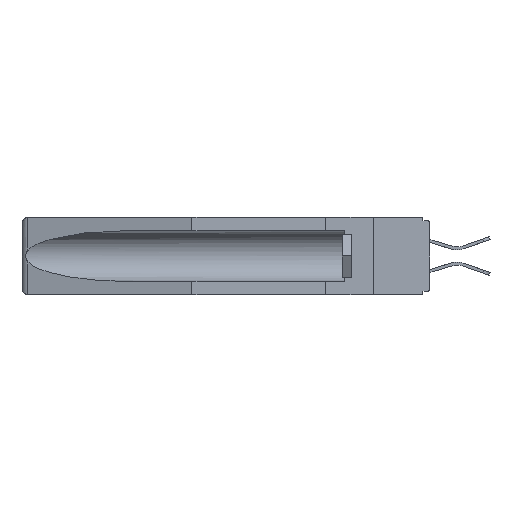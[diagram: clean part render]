
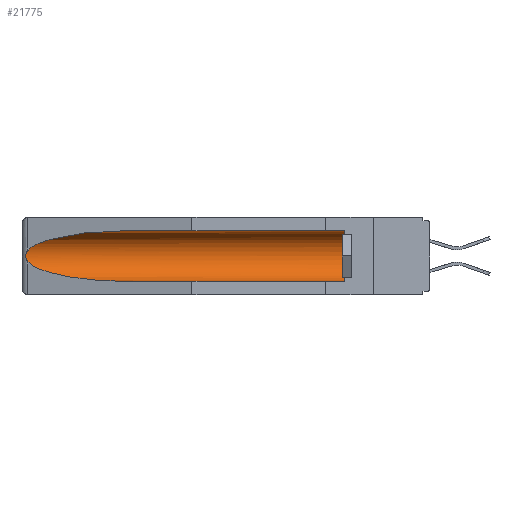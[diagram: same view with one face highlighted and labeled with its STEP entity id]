
A CAD part, left-side view. The second image highlights one B-rep face of the part: STEP entity #21775.
In plain terms, the highlighted cylindrical face has radius 2.857 mm (diameter 5.715 mm), a partial arc.
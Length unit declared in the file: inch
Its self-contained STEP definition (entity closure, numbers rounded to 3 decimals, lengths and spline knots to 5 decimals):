
#43 = CARTESIAN_POINT ( 'NONE',  ( 0.155, 1.07973, -0.284 ) ) ;
#302 = CARTESIAN_POINT ( 'NONE',  ( 0.155, 0.126, -0.284 ) ) ;
#772 = DIRECTION ( 'NONE',  ( 0., 1., 0. ) ) ;
#1684 = CARTESIAN_POINT ( 'NONE',  ( 0.155, 0.126, -0.059 ) ) ;
#1730 = DIRECTION ( 'NONE',  ( 0., 0., 1. ) ) ;
#1819 = CARTESIAN_POINT ( 'NONE',  ( 0.25451, 1.48313, -0.24835 ) ) ;
#1913 = EDGE_CURVE ( 'NONE', #20952, #2292, #11768, .T. ) ;
#1987 = CARTESIAN_POINT ( 'NONE',  ( 0.26537, 1.52718, -0.19328 ) ) ;
#2146 = CARTESIAN_POINT ( 'NONE',  ( 0.26654, 1.53092, -0.15636 ) ) ;
#2292 = VERTEX_POINT ( 'NONE', #5567 ) ;
#2320 = EDGE_CURVE ( 'NONE', #10931, #20379, #12574, .T. ) ;
#2495 = VECTOR ( 'NONE', #7397, 39.37008 ) ;
#3143 = CARTESIAN_POINT ( 'NONE',  ( 0.26537, 1.52718, -0.19328 ) ) ;
#3879 = CARTESIAN_POINT ( 'NONE',  ( 0.2675, 1.53308, -0.16763 ) ) ;
#3963 = CARTESIAN_POINT ( 'NONE',  ( 0.2673, 1.5327, -0.16383 ) ) ;
#4020 = CARTESIAN_POINT ( 'NONE',  ( 0.155, -0.30754, -0.284 ) ) ;
#4462 = CARTESIAN_POINT ( 'NONE',  ( 0.155, 1.07973, -0.059 ) ) ;
#4467 = ORIENTED_EDGE ( 'NONE', *, *, #15019, .T. ) ;
#4887 = ORIENTED_EDGE ( 'NONE', *, *, #8083, .T. ) ;
#5567 = CARTESIAN_POINT ( 'NONE',  ( 0.26537, 1.52718, -0.19328 ) ) ;
#5829 = CARTESIAN_POINT ( 'NONE',  ( 0.26597, 1.5296, -0.19026 ) ) ;
#6010 = CARTESIAN_POINT ( 'NONE',  ( 0.21114, 1.30732, -0.059 ) ) ;
#6407 = EDGE_LOOP ( 'NONE', ( #17727, #14989, #4467, #18095, #15805, #4887 ) ) ;
#7132 = CARTESIAN_POINT ( 'NONE',  ( 0.155, 1.07973, -0.059 ) ) ;
#7335 = CARTESIAN_POINT ( 'NONE',  ( 0.21114, 1.30732, -0.284 ) ) ;
#7397 = DIRECTION ( 'NONE',  ( 0., 1., 0. ) ) ;
#7503 = CARTESIAN_POINT ( 'NONE',  ( 0.26655, 1.53094, -0.18657 ) ) ;
#8083 = EDGE_CURVE ( 'NONE', #20379, #16421, #15592, .T. ) ;
#9657 = CARTESIAN_POINT ( 'NONE',  ( 0.155, -0.30754, -0.059 ) ) ;
#10472 = AXIS2_PLACEMENT_3D ( 'NONE', #23504, #12656, #1730 ) ;
#10912 = AXIS2_PLACEMENT_3D ( 'NONE', #21852, #20185, #22017 ) ;
#10931 = VERTEX_POINT ( 'NONE', #302 ) ;
#11586 = EDGE_CURVE ( 'NONE', #16421, #20952, #13906, .T. ) ;
#11768 = B_SPLINE_CURVE_WITH_KNOTS ( 'NONE', 3,
 ( #12844, #13071, #2146, #3963, #3879, #18599, #16687, #7503, #5829, #1987 ),
 .UNSPECIFIED., .F., .F.,
 ( 4, 2, 2, 2, 4 ),
 ( 0., 0.00029, 0.00058, 0.00087, 0.00117 ),
 .UNSPECIFIED. ) ;
#12211 = CARTESIAN_POINT ( 'NONE',  ( 0.155, 1.07973, -0.284 ) ) ;
#12574 = CIRCLE ( 'NONE', #10472, 0.1125 ) ;
#12656 = DIRECTION ( 'NONE',  ( 0., -1., 0. ) ) ;
#12844 = CARTESIAN_POINT ( 'NONE',  ( 0.26537, 1.52718, -0.14972 ) ) ;
#13071 = CARTESIAN_POINT ( 'NONE',  ( 0.26597, 1.52961, -0.15275 ) ) ;
#13388 = CARTESIAN_POINT ( 'NONE',  ( 0.26537, 1.52718, -0.14972 ) ) ;
#13906 =( BOUNDED_CURVE ( )  B_SPLINE_CURVE ( 3, ( #4462, #6010, #19001, #13388 ),
 .UNSPECIFIED., .F., .F. ) 
 B_SPLINE_CURVE_WITH_KNOTS ( ( 4, 4 ),
 ( 4.71239, 6.08839 ),
 .UNSPECIFIED. ) 
 CURVE ( )  GEOMETRIC_REPRESENTATION_ITEM ( )  RATIONAL_B_SPLINE_CURVE ( ( 1., 0.848, 0.848, 1. ) ) 
 REPRESENTATION_ITEM ( '' )  );
#14989 = ORIENTED_EDGE ( 'NONE', *, *, #1913, .T. ) ;
#15019 = EDGE_CURVE ( 'NONE', #2292, #20888, #16364, .T. ) ;
#15592 = LINE ( 'NONE', #9657, #22140 ) ;
#15805 = ORIENTED_EDGE ( 'NONE', *, *, #2320, .T. ) ;
#16364 =( BOUNDED_CURVE ( )  B_SPLINE_CURVE ( 3, ( #3143, #1819, #7335, #43 ),
 .UNSPECIFIED., .F., .F. ) 
 B_SPLINE_CURVE_WITH_KNOTS ( ( 4, 4 ),
 ( 0.1948, 1.5708 ),
 .UNSPECIFIED. ) 
 CURVE ( )  GEOMETRIC_REPRESENTATION_ITEM ( )  RATIONAL_B_SPLINE_CURVE ( ( 1., 0.848, 0.848, 1. ) ) 
 REPRESENTATION_ITEM ( '' )  );
#16401 = FACE_OUTER_BOUND ( 'NONE', #6407, .T. ) ;
#16421 = VERTEX_POINT ( 'NONE', #7132 ) ;
#16671 = CYLINDRICAL_SURFACE ( 'NONE', #10912, 0.1125 ) ;
#16687 = CARTESIAN_POINT ( 'NONE',  ( 0.2673, 1.53269, -0.17917 ) ) ;
#16996 = LINE ( 'NONE', #4020, #2495 ) ;
#17727 = ORIENTED_EDGE ( 'NONE', *, *, #11586, .T. ) ;
#18095 = ORIENTED_EDGE ( 'NONE', *, *, #22690, .F. ) ;
#18599 = CARTESIAN_POINT ( 'NONE',  ( 0.2675, 1.53308, -0.17534 ) ) ;
#19001 = CARTESIAN_POINT ( 'NONE',  ( 0.25451, 1.48313, -0.09465 ) ) ;
#20185 = DIRECTION ( 'NONE',  ( 0., 1., 0. ) ) ;
#20379 = VERTEX_POINT ( 'NONE', #1684 ) ;
#20888 = VERTEX_POINT ( 'NONE', #12211 ) ;
#20952 = VERTEX_POINT ( 'NONE', #23367 ) ;
#21775 = ADVANCED_FACE ( 'NONE', ( #16401 ), #16671, .F. ) ;
#21852 = CARTESIAN_POINT ( 'NONE',  ( 0.155, -0.30754, -0.1715 ) ) ;
#22017 = DIRECTION ( 'NONE',  ( 0., 0., 1. ) ) ;
#22140 = VECTOR ( 'NONE', #772, 39.37008 ) ;
#22690 = EDGE_CURVE ( 'NONE', #10931, #20888, #16996, .T. ) ;
#23367 = CARTESIAN_POINT ( 'NONE',  ( 0.26537, 1.52718, -0.14972 ) ) ;
#23504 = CARTESIAN_POINT ( 'NONE',  ( 0.155, 0.126, -0.1715 ) ) ;
